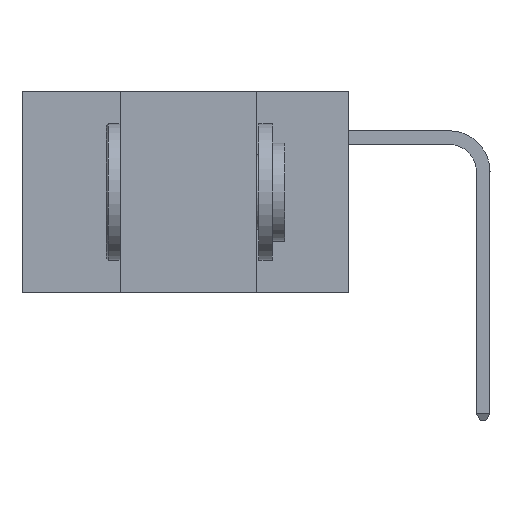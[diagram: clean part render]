
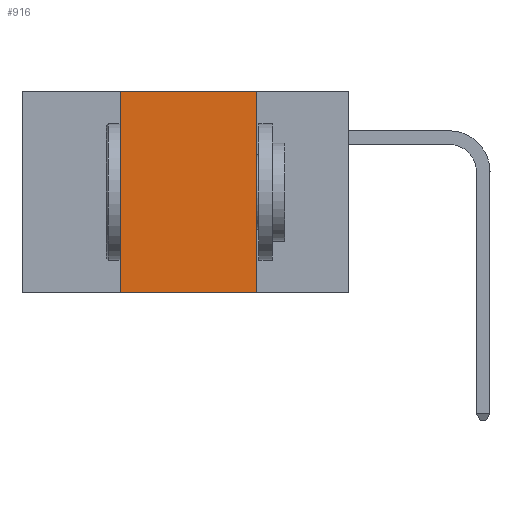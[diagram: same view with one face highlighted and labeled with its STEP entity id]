
A CAD part, left-side view. The second image highlights one B-rep face of the part: STEP entity #916.
In plain terms, the highlighted planar face has unit normal (-1, 0, 0).
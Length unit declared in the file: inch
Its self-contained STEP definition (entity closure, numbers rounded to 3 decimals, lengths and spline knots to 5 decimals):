
#234 = EDGE_CURVE ( 'NONE', #12507, #12435, #13275, .T. ) ;
#916 = ADVANCED_FACE ( 'NONE', ( #9887 ), #3469, .F. ) ;
#938 = CARTESIAN_POINT ( 'NONE',  ( 0., 0.6, 0. ) ) ;
#1020 = CARTESIAN_POINT ( 'NONE',  ( 0., 0.17, 0. ) ) ;
#1026 = ORIENTED_EDGE ( 'NONE', *, *, #8214, .F. ) ;
#2544 = CARTESIAN_POINT ( 'NONE',  ( 0., 0.42, 0. ) ) ;
#3469 = PLANE ( 'NONE',  #10035 ) ;
#3540 = DIRECTION ( 'NONE',  ( 0., -1., 0. ) ) ;
#3679 = ORIENTED_EDGE ( 'NONE', *, *, #234, .T. ) ;
#4053 = CARTESIAN_POINT ( 'NONE',  ( 0., 0.17, 0. ) ) ;
#5383 = VERTEX_POINT ( 'NONE', #1020 ) ;
#5592 = LINE ( 'NONE', #2544, #10988 ) ;
#5956 = CARTESIAN_POINT ( 'NONE',  ( 0., 0.6, 0. ) ) ;
#6241 = CARTESIAN_POINT ( 'NONE',  ( 0., 0.17, -0.37 ) ) ;
#7267 = VECTOR ( 'NONE', #13892, 39.37008 ) ;
#7270 = ORIENTED_EDGE ( 'NONE', *, *, #9929, .F. ) ;
#7989 = DIRECTION ( 'NONE',  ( 1., 0., 0. ) ) ;
#8099 = LINE ( 'NONE', #938, #7267 ) ;
#8214 = EDGE_CURVE ( 'NONE', #12507, #10759, #5592, .T. ) ;
#8762 = CARTESIAN_POINT ( 'NONE',  ( 0., 0.6, -0.37 ) ) ;
#9887 = FACE_OUTER_BOUND ( 'NONE', #12115, .T. ) ;
#9913 = VECTOR ( 'NONE', #10646, 39.37008 ) ;
#9929 = EDGE_CURVE ( 'NONE', #5383, #12435, #12107, .T. ) ;
#10035 = AXIS2_PLACEMENT_3D ( 'NONE', #5956, #7989, #11234 ) ;
#10297 = CARTESIAN_POINT ( 'NONE',  ( 0., 0.42, 0. ) ) ;
#10646 = DIRECTION ( 'NONE',  ( 0., 0., -1. ) ) ;
#10759 = VERTEX_POINT ( 'NONE', #10297 ) ;
#10988 = VECTOR ( 'NONE', #11145, 39.37008 ) ;
#11145 = DIRECTION ( 'NONE',  ( 0., 0., 1. ) ) ;
#11234 = DIRECTION ( 'NONE',  ( 0., 0., -1. ) ) ;
#11585 = VECTOR ( 'NONE', #3540, 39.37008 ) ;
#12107 = LINE ( 'NONE', #4053, #9913 ) ;
#12115 = EDGE_LOOP ( 'NONE', ( #7270, #12363, #1026, #3679 ) ) ;
#12363 = ORIENTED_EDGE ( 'NONE', *, *, #13855, .F. ) ;
#12435 = VERTEX_POINT ( 'NONE', #6241 ) ;
#12507 = VERTEX_POINT ( 'NONE', #13888 ) ;
#13275 = LINE ( 'NONE', #8762, #11585 ) ;
#13855 = EDGE_CURVE ( 'NONE', #10759, #5383, #8099, .T. ) ;
#13888 = CARTESIAN_POINT ( 'NONE',  ( 0., 0.42, -0.37 ) ) ;
#13892 = DIRECTION ( 'NONE',  ( 0., -1., 0. ) ) ;
